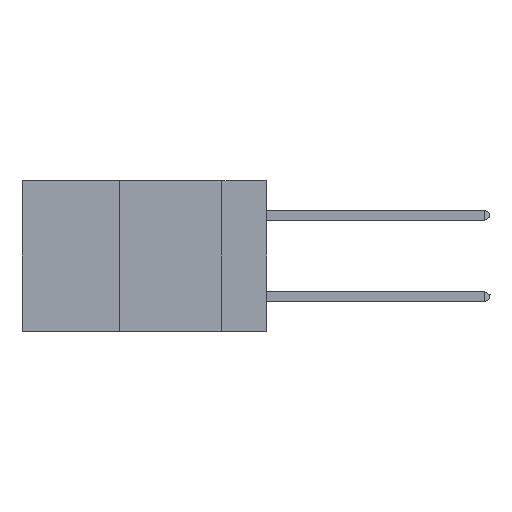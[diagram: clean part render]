
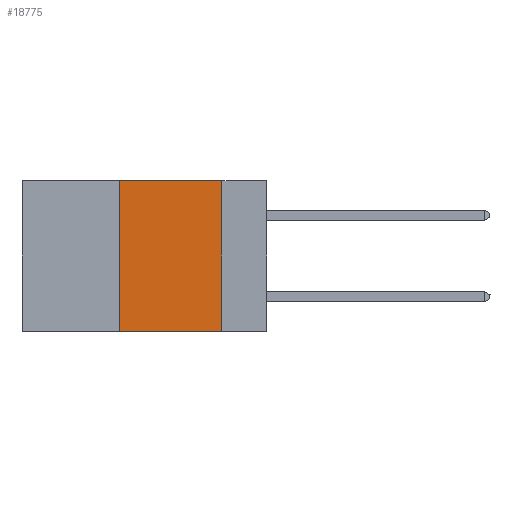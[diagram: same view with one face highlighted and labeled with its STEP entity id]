
A CAD part, left-side view. The second image highlights one B-rep face of the part: STEP entity #18775.
In plain terms, the highlighted planar face has unit normal (-1, 0, 0).
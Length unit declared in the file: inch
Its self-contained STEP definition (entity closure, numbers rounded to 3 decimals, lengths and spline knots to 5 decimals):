
#604 = VECTOR ( 'NONE', #13189, 39.37008 ) ;
#2122 = LINE ( 'NONE', #5547, #19910 ) ;
#2152 = VECTOR ( 'NONE', #7137, 39.37008 ) ;
#3573 = LINE ( 'NONE', #15676, #9282 ) ;
#4501 = DIRECTION ( 'NONE',  ( 1., 0., 0. ) ) ;
#5240 = LINE ( 'NONE', #18319, #604 ) ;
#5547 = CARTESIAN_POINT ( 'NONE',  ( 0., 0.6, 0. ) ) ;
#5700 = CARTESIAN_POINT ( 'NONE',  ( 0., 0.36, -0.37 ) ) ;
#6721 = DIRECTION ( 'NONE',  ( 0., 0., -1. ) ) ;
#7137 = DIRECTION ( 'NONE',  ( 0., -1., 0. ) ) ;
#8265 = ORIENTED_EDGE ( 'NONE', *, *, #19707, .F. ) ;
#8711 = DIRECTION ( 'NONE',  ( 0., 0., -1. ) ) ;
#8930 = CARTESIAN_POINT ( 'NONE',  ( 0., 0.6, -0.37 ) ) ;
#9282 = VECTOR ( 'NONE', #8711, 39.37008 ) ;
#10425 = VERTEX_POINT ( 'NONE', #17416 ) ;
#10784 = ORIENTED_EDGE ( 'NONE', *, *, #18700, .F. ) ;
#10860 = EDGE_CURVE ( 'NONE', #17266, #21919, #2122, .T. ) ;
#12557 = DIRECTION ( 'NONE',  ( 0., -1., 0. ) ) ;
#12628 = CARTESIAN_POINT ( 'NONE',  ( 0., 0.11, 0. ) ) ;
#13189 = DIRECTION ( 'NONE',  ( 0., 0., 1. ) ) ;
#13988 = FACE_OUTER_BOUND ( 'NONE', #14981, .T. ) ;
#14480 = CARTESIAN_POINT ( 'NONE',  ( 0., 0.36, 0. ) ) ;
#14981 = EDGE_LOOP ( 'NONE', ( #8265, #21064, #10784, #20545 ) ) ;
#15676 = CARTESIAN_POINT ( 'NONE',  ( 0., 0.11, 0. ) ) ;
#15873 = EDGE_CURVE ( 'NONE', #20557, #10425, #17723, .T. ) ;
#16937 = AXIS2_PLACEMENT_3D ( 'NONE', #20233, #4501, #6721 ) ;
#17266 = VERTEX_POINT ( 'NONE', #14480 ) ;
#17416 = CARTESIAN_POINT ( 'NONE',  ( 0., 0.11, -0.37 ) ) ;
#17723 = LINE ( 'NONE', #8930, #2152 ) ;
#18319 = CARTESIAN_POINT ( 'NONE',  ( 0., 0.36, 0. ) ) ;
#18700 = EDGE_CURVE ( 'NONE', #20557, #17266, #5240, .T. ) ;
#18775 = ADVANCED_FACE ( 'NONE', ( #13988 ), #20156, .F. ) ;
#19707 = EDGE_CURVE ( 'NONE', #21919, #10425, #3573, .T. ) ;
#19910 = VECTOR ( 'NONE', #12557, 39.37008 ) ;
#20156 = PLANE ( 'NONE',  #16937 ) ;
#20233 = CARTESIAN_POINT ( 'NONE',  ( 0., 0.6, 0. ) ) ;
#20545 = ORIENTED_EDGE ( 'NONE', *, *, #15873, .T. ) ;
#20557 = VERTEX_POINT ( 'NONE', #5700 ) ;
#21064 = ORIENTED_EDGE ( 'NONE', *, *, #10860, .F. ) ;
#21919 = VERTEX_POINT ( 'NONE', #12628 ) ;
